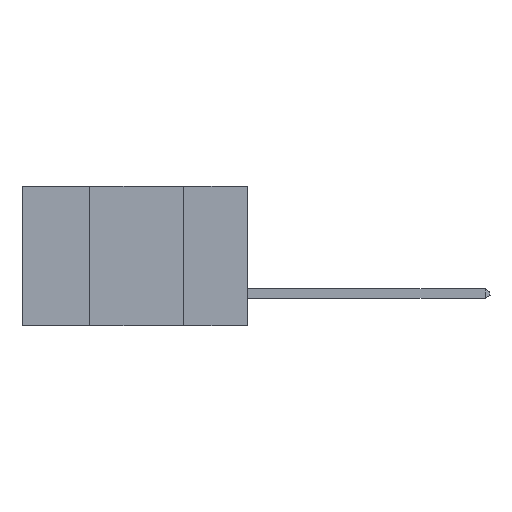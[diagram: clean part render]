
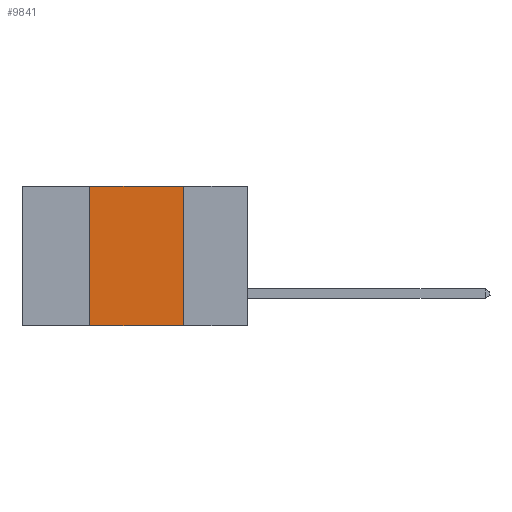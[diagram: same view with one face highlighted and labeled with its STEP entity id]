
A CAD part, left-side view. The second image highlights one B-rep face of the part: STEP entity #9841.
In plain terms, the highlighted planar face has unit normal (-1, 0, 0).
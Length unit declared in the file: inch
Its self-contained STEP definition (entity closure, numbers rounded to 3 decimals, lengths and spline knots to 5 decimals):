
#224 = DIRECTION ( 'NONE',  ( 1., 0., 0. ) ) ;
#362 = DIRECTION ( 'NONE',  ( 0., -1., 0. ) ) ;
#1414 = EDGE_CURVE ( 'NONE', #9810, #17473, #8799, .T. ) ;
#1495 = ORIENTED_EDGE ( 'NONE', *, *, #12218, .F. ) ;
#2693 = VERTEX_POINT ( 'NONE', #14582 ) ;
#2952 = ORIENTED_EDGE ( 'NONE', *, *, #11161, .F. ) ;
#3699 = DIRECTION ( 'NONE',  ( 0., -1., 0. ) ) ;
#4145 = CARTESIAN_POINT ( 'NONE',  ( 0., 0.6, 0. ) ) ;
#4947 = CARTESIAN_POINT ( 'NONE',  ( 0., 0.42, 0. ) ) ;
#5179 = LINE ( 'NONE', #4947, #7397 ) ;
#5957 = CARTESIAN_POINT ( 'NONE',  ( 0., 0.17, 0. ) ) ;
#6489 = DIRECTION ( 'NONE',  ( 0., 0., 1. ) ) ;
#7127 = EDGE_CURVE ( 'NONE', #7521, #17473, #13141, .T. ) ;
#7153 = DIRECTION ( 'NONE',  ( 0., 0., -1. ) ) ;
#7397 = VECTOR ( 'NONE', #6489, 39.37008 ) ;
#7521 = VERTEX_POINT ( 'NONE', #9998 ) ;
#8799 = LINE ( 'NONE', #5957, #15487 ) ;
#8876 = CARTESIAN_POINT ( 'NONE',  ( 0., 0.6, -0.37 ) ) ;
#9777 = PLANE ( 'NONE',  #16556 ) ;
#9810 = VERTEX_POINT ( 'NONE', #10971 ) ;
#9841 = ADVANCED_FACE ( 'NONE', ( #17755 ), #9777, .F. ) ;
#9998 = CARTESIAN_POINT ( 'NONE',  ( 0., 0.42, -0.37 ) ) ;
#10760 = CARTESIAN_POINT ( 'NONE',  ( 0., 0.6, 0. ) ) ;
#10897 = VECTOR ( 'NONE', #362, 39.37008 ) ;
#10971 = CARTESIAN_POINT ( 'NONE',  ( 0., 0.17, 0. ) ) ;
#11161 = EDGE_CURVE ( 'NONE', #2693, #9810, #11886, .T. ) ;
#11751 = EDGE_LOOP ( 'NONE', ( #11869, #2952, #1495, #16936 ) ) ;
#11869 = ORIENTED_EDGE ( 'NONE', *, *, #1414, .F. ) ;
#11886 = LINE ( 'NONE', #10760, #17278 ) ;
#12218 = EDGE_CURVE ( 'NONE', #7521, #2693, #5179, .T. ) ;
#12931 = DIRECTION ( 'NONE',  ( 0., 0., -1. ) ) ;
#13141 = LINE ( 'NONE', #8876, #10897 ) ;
#13783 = CARTESIAN_POINT ( 'NONE',  ( 0., 0.17, -0.37 ) ) ;
#14582 = CARTESIAN_POINT ( 'NONE',  ( 0., 0.42, 0. ) ) ;
#15487 = VECTOR ( 'NONE', #7153, 39.37008 ) ;
#16556 = AXIS2_PLACEMENT_3D ( 'NONE', #4145, #224, #12931 ) ;
#16936 = ORIENTED_EDGE ( 'NONE', *, *, #7127, .T. ) ;
#17278 = VECTOR ( 'NONE', #3699, 39.37008 ) ;
#17473 = VERTEX_POINT ( 'NONE', #13783 ) ;
#17755 = FACE_OUTER_BOUND ( 'NONE', #11751, .T. ) ;
